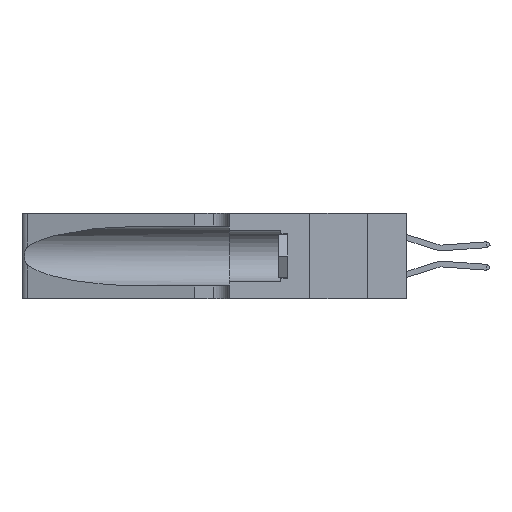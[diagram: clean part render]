
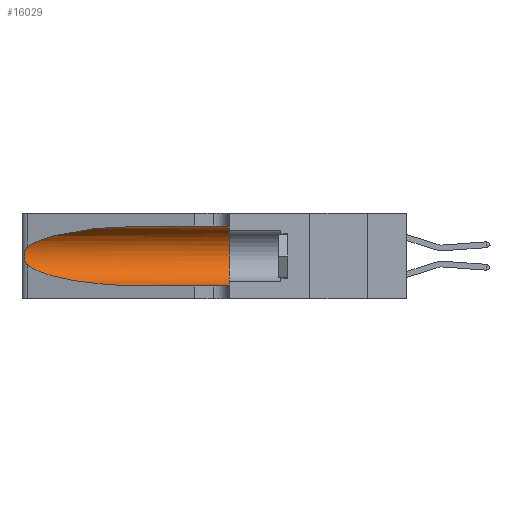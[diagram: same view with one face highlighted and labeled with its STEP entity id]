
A CAD part, left-side view. The second image highlights one B-rep face of the part: STEP entity #16029.
In plain terms, the highlighted cylindrical face has radius 3.308 mm (diameter 6.617 mm), a partial arc.
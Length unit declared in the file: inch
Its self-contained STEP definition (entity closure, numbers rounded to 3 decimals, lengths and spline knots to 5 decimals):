
#163 = CARTESIAN_POINT ( 'NONE',  ( 0.1305, 0.35, 0.185 ) ) ;
#214 = CARTESIAN_POINT ( 'NONE',  ( 0.25789, 1.23486, 0.15765 ) ) ;
#586 = CARTESIAN_POINT ( 'NONE',  ( 0.25854, 1.2359, 0.20912 ) ) ;
#688 = CARTESIAN_POINT ( 'NONE',  ( 0.25487, 1.22718, 0.14631 ) ) ;
#1224 = DIRECTION ( 'NONE',  ( 0., 0., -1. ) ) ;
#1590 = CARTESIAN_POINT ( 'NONE',  ( 0.18966, 0.96281, 0.05475 ) ) ;
#2145 = EDGE_CURVE ( 'NONE', #9796, #5741, #10117, .T. ) ;
#2269 = CARTESIAN_POINT ( 'NONE',  ( 0.1305, 0.35, 0.05475 ) ) ;
#2670 = CARTESIAN_POINT ( 'NONE',  ( 0.25639, 1.23186, 0.15144 ) ) ;
#2742 = CARTESIAN_POINT ( 'NONE',  ( 0.1305, 1.61858, 0.05475 ) ) ;
#3756 = CARTESIAN_POINT ( 'NONE',  ( 0.1305, 0.72297, 0.05475 ) ) ;
#4575 = CARTESIAN_POINT ( 'NONE',  ( 0.26075, 1.23896, 0.19203 ) ) ;
#4762 = CARTESIAN_POINT ( 'NONE',  ( 0.25487, 1.22718, 0.14631 ) ) ;
#4950 = CARTESIAN_POINT ( 'NONE',  ( 0.26017, 1.23833, 0.17102 ) ) ;
#5107 = CARTESIAN_POINT ( 'NONE',  ( 0.1305, 1.61858, 0.185 ) ) ;
#5479 = VERTEX_POINT ( 'NONE', #16424 ) ;
#5741 = VERTEX_POINT ( 'NONE', #21272 ) ;
#6328 = ORIENTED_EDGE ( 'NONE', *, *, #20009, .F. ) ;
#6629 = DIRECTION ( 'NONE',  ( 0., 1., 0. ) ) ;
#6969 = CARTESIAN_POINT ( 'NONE',  ( 0.25555, 1.22994, 0.2215 ) ) ;
#7014 = EDGE_CURVE ( 'NONE', #14798, #25234, #24776, .T. ) ;
#7465 =( BOUNDED_CURVE ( )  B_SPLINE_CURVE ( 3, ( #9685, #9486, #11673, #16063 ),
 .UNSPECIFIED., .F., .F. ) 
 B_SPLINE_CURVE_WITH_KNOTS ( ( 4, 4 ),
 ( 1.5708, 2.84003 ),
 .UNSPECIFIED. ) 
 CURVE ( )  GEOMETRIC_REPRESENTATION_ITEM ( )  RATIONAL_B_SPLINE_CURVE ( ( 1., 0.87, 0.87, 1. ) ) 
 REPRESENTATION_ITEM ( '' )  );
#7768 = ORIENTED_EDGE ( 'NONE', *, *, #19689, .T. ) ;
#9039 = CARTESIAN_POINT ( 'NONE',  ( 0.25555, 1.22993, 0.14849 ) ) ;
#9408 = CARTESIAN_POINT ( 'NONE',  ( 0.25639, 1.23184, 0.21858 ) ) ;
#9486 = CARTESIAN_POINT ( 'NONE',  ( 0.18966, 0.96281, 0.31525 ) ) ;
#9685 = CARTESIAN_POINT ( 'NONE',  ( 0.1305, 0.72297, 0.31525 ) ) ;
#9796 = VERTEX_POINT ( 'NONE', #688 ) ;
#10117 =( BOUNDED_CURVE ( )  B_SPLINE_CURVE ( 3, ( #27669, #14687, #1590, #3756 ),
 .UNSPECIFIED., .F., .F. ) 
 B_SPLINE_CURVE_WITH_KNOTS ( ( 4, 4 ),
 ( 3.44316, 4.71239 ),
 .UNSPECIFIED. ) 
 CURVE ( )  GEOMETRIC_REPRESENTATION_ITEM ( )  RATIONAL_B_SPLINE_CURVE ( ( 1., 0.87, 0.87, 1. ) ) 
 REPRESENTATION_ITEM ( '' )  );
#10257 = VERTEX_POINT ( 'NONE', #2269 ) ;
#11673 = CARTESIAN_POINT ( 'NONE',  ( 0.2373, 1.15595, 0.28018 ) ) ;
#11814 = ORIENTED_EDGE ( 'NONE', *, *, #17155, .T. ) ;
#13693 = CARTESIAN_POINT ( 'NONE',  ( 0.26075, 1.23896, 0.178 ) ) ;
#14687 = CARTESIAN_POINT ( 'NONE',  ( 0.2373, 1.15595, 0.08982 ) ) ;
#14798 = VERTEX_POINT ( 'NONE', #27079 ) ;
#15350 = ORIENTED_EDGE ( 'NONE', *, *, #7014, .F. ) ;
#16029 = ADVANCED_FACE ( 'NONE', ( #17607 ), #28150, .F. ) ;
#16063 = CARTESIAN_POINT ( 'NONE',  ( 0.25487, 1.22718, 0.22369 ) ) ;
#16401 = B_SPLINE_CURVE_WITH_KNOTS ( 'NONE', 3,
 ( #26685, #6969, #9408, #22191, #586, #18016, #4575, #13693, #4950, #26772, #214, #2670, #9039, #4762 ),
 .UNSPECIFIED., .F., .F.,
 ( 4, 2, 2, 2, 2, 2, 4 ),
 ( 0., 0.00027, 0.00053, 0.00107, 0.0016, 0.00187, 0.00214 ),
 .UNSPECIFIED. ) ;
#16424 = CARTESIAN_POINT ( 'NONE',  ( 0.25487, 1.22718, 0.22369 ) ) ;
#16665 = DIRECTION ( 'NONE',  ( 0., -1., 0. ) ) ;
#16778 = ORIENTED_EDGE ( 'NONE', *, *, #20825, .T. ) ;
#17155 = EDGE_CURVE ( 'NONE', #14798, #5479, #7465, .T. ) ;
#17607 = FACE_OUTER_BOUND ( 'NONE', #21984, .T. ) ;
#17653 = VECTOR ( 'NONE', #16665, 39.37008 ) ;
#17684 = DIRECTION ( 'NONE',  ( 0., 0., 1. ) ) ;
#17987 = DIRECTION ( 'NONE',  ( 0., -1., 0. ) ) ;
#18016 = CARTESIAN_POINT ( 'NONE',  ( 0.26018, 1.23835, 0.19895 ) ) ;
#18258 = AXIS2_PLACEMENT_3D ( 'NONE', #5107, #26916, #1224 ) ;
#19689 = EDGE_CURVE ( 'NONE', #5741, #10257, #27680, .T. ) ;
#19954 = ORIENTED_EDGE ( 'NONE', *, *, #2145, .T. ) ;
#20009 = EDGE_CURVE ( 'NONE', #25234, #10257, #24930, .T. ) ;
#20825 = EDGE_CURVE ( 'NONE', #5479, #9796, #16401, .T. ) ;
#20977 = CARTESIAN_POINT ( 'NONE',  ( 0.1305, 1.61858, 0.31525 ) ) ;
#21272 = CARTESIAN_POINT ( 'NONE',  ( 0.1305, 0.72297, 0.05475 ) ) ;
#21984 = EDGE_LOOP ( 'NONE', ( #11814, #16778, #19954, #7768, #6328, #15350 ) ) ;
#22191 = CARTESIAN_POINT ( 'NONE',  ( 0.25787, 1.23484, 0.2124 ) ) ;
#24012 = AXIS2_PLACEMENT_3D ( 'NONE', #163, #6629, #17684 ) ;
#24602 = VECTOR ( 'NONE', #17987, 39.37008 ) ;
#24776 = LINE ( 'NONE', #20977, #17653 ) ;
#24930 = CIRCLE ( 'NONE', #24012, 0.13025 ) ;
#25077 = CARTESIAN_POINT ( 'NONE',  ( 0.1305, 0.35, 0.31525 ) ) ;
#25234 = VERTEX_POINT ( 'NONE', #25077 ) ;
#26685 = CARTESIAN_POINT ( 'NONE',  ( 0.25487, 1.22718, 0.22369 ) ) ;
#26772 = CARTESIAN_POINT ( 'NONE',  ( 0.25856, 1.23593, 0.16098 ) ) ;
#26916 = DIRECTION ( 'NONE',  ( 0., -1., 0. ) ) ;
#27079 = CARTESIAN_POINT ( 'NONE',  ( 0.1305, 0.72297, 0.31525 ) ) ;
#27669 = CARTESIAN_POINT ( 'NONE',  ( 0.25487, 1.22718, 0.14631 ) ) ;
#27680 = LINE ( 'NONE', #2742, #24602 ) ;
#28150 = CYLINDRICAL_SURFACE ( 'NONE', #18258, 0.13025 ) ;
